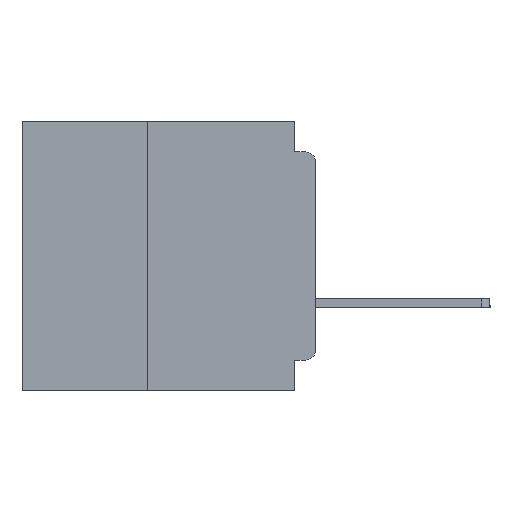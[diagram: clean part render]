
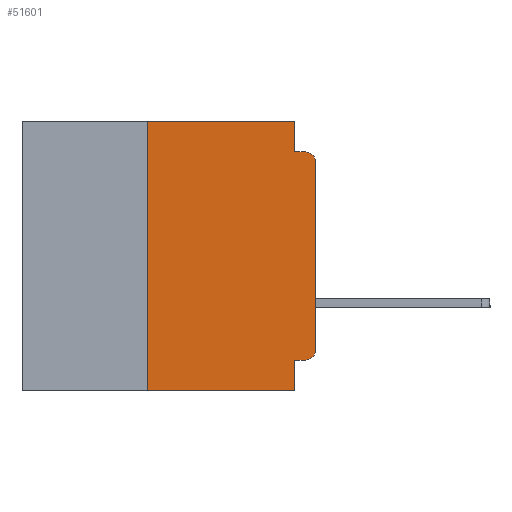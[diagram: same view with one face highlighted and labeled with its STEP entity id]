
A CAD part, left-side view. The second image highlights one B-rep face of the part: STEP entity #51601.
In plain terms, the highlighted planar face has unit normal (-1, 0, 0).
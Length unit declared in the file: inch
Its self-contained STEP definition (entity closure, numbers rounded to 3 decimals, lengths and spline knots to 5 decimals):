
#719 = CARTESIAN_POINT ( 'NONE',  ( 0., 0.031, 0. ) ) ;
#897 = LINE ( 'NONE', #25020, #22714 ) ;
#925 = EDGE_CURVE ( 'NONE', #34286, #8893, #15432, .T. ) ;
#1005 = DIRECTION ( 'NONE',  ( 0., 0., -1. ) ) ;
#1437 = ORIENTED_EDGE ( 'NONE', *, *, #4364, .F. ) ;
#3065 = LINE ( 'NONE', #24203, #42566 ) ;
#4200 = VERTEX_POINT ( 'NONE', #6494 ) ;
#4231 = ORIENTED_EDGE ( 'NONE', *, *, #51939, .F. ) ;
#4238 = DIRECTION ( 'NONE',  ( 0., -1., 0. ) ) ;
#4364 = EDGE_CURVE ( 'NONE', #16889, #38575, #39948, .T. ) ;
#4849 = CARTESIAN_POINT ( 'NONE',  ( 0., 0.031, -0.355 ) ) ;
#5773 = CARTESIAN_POINT ( 'NONE',  ( 0., 0., -0.06 ) ) ;
#6494 = CARTESIAN_POINT ( 'NONE',  ( 0., 0.015, -0.355 ) ) ;
#6663 = CARTESIAN_POINT ( 'NONE',  ( 0., 0.015, -0.06 ) ) ;
#6744 = LINE ( 'NONE', #23052, #37962 ) ;
#8608 = ORIENTED_EDGE ( 'NONE', *, *, #21193, .F. ) ;
#8769 = DIRECTION ( 'NONE',  ( 0., 0., 1. ) ) ;
#8893 = VERTEX_POINT ( 'NONE', #5773 ) ;
#9596 = CARTESIAN_POINT ( 'NONE',  ( 0., 0., 0. ) ) ;
#10766 = DIRECTION ( 'NONE',  ( 0., 0., -1. ) ) ;
#10868 = DIRECTION ( 'NONE',  ( -1., 0., 0. ) ) ;
#13558 = PLANE ( 'NONE',  #44437 ) ;
#13736 = LINE ( 'NONE', #24589, #24548 ) ;
#14921 = CIRCLE ( 'NONE', #21644, 0.015 ) ;
#15432 = LINE ( 'NONE', #9596, #22434 ) ;
#16889 = VERTEX_POINT ( 'NONE', #21702 ) ;
#17095 = VERTEX_POINT ( 'NONE', #23110 ) ;
#17670 = CARTESIAN_POINT ( 'NONE',  ( 0., 0.437, 0. ) ) ;
#17937 = ORIENTED_EDGE ( 'NONE', *, *, #28486, .F. ) ;
#19369 = CARTESIAN_POINT ( 'NONE',  ( 0., 0.25, 0. ) ) ;
#19868 = VECTOR ( 'NONE', #26842, 39.37008 ) ;
#20534 = CARTESIAN_POINT ( 'NONE',  ( 0., 0.25, -0.4 ) ) ;
#21193 = EDGE_CURVE ( 'NONE', #38575, #17095, #13736, .T. ) ;
#21644 = AXIS2_PLACEMENT_3D ( 'NONE', #35237, #10868, #39339 ) ;
#21702 = CARTESIAN_POINT ( 'NONE',  ( 0., 0.031, 0. ) ) ;
#21763 = DIRECTION ( 'NONE',  ( 1., 0., 0. ) ) ;
#22224 = ORIENTED_EDGE ( 'NONE', *, *, #41233, .T. ) ;
#22434 = VECTOR ( 'NONE', #8769, 39.37008 ) ;
#22470 = VERTEX_POINT ( 'NONE', #35575 ) ;
#22714 = VECTOR ( 'NONE', #49220, 39.37008 ) ;
#22882 = DIRECTION ( 'NONE',  ( 0., -1., 0. ) ) ;
#23052 = CARTESIAN_POINT ( 'NONE',  ( 0., 0.25, -0.4 ) ) ;
#23110 = CARTESIAN_POINT ( 'NONE',  ( 0., 0.015, -0.045 ) ) ;
#24203 = CARTESIAN_POINT ( 'NONE',  ( 0., 0., -0.355 ) ) ;
#24548 = VECTOR ( 'NONE', #4238, 39.37008 ) ;
#24589 = CARTESIAN_POINT ( 'NONE',  ( 0., 0., -0.045 ) ) ;
#25020 = CARTESIAN_POINT ( 'NONE',  ( 0., 0.437, -0.4 ) ) ;
#26067 = CARTESIAN_POINT ( 'NONE',  ( 0., 0., -0.34 ) ) ;
#26842 = DIRECTION ( 'NONE',  ( 0., 0., -1. ) ) ;
#28486 = EDGE_CURVE ( 'NONE', #35726, #16889, #41700, .T. ) ;
#28752 = VERTEX_POINT ( 'NONE', #20534 ) ;
#30394 = EDGE_CURVE ( 'NONE', #4200, #34286, #14921, .T. ) ;
#30603 = FACE_OUTER_BOUND ( 'NONE', #38740, .T. ) ;
#31379 = VERTEX_POINT ( 'NONE', #4849 ) ;
#31472 = ORIENTED_EDGE ( 'NONE', *, *, #925, .T. ) ;
#31729 = CIRCLE ( 'NONE', #39389, 0.015 ) ;
#32222 = VECTOR ( 'NONE', #22882, 39.37008 ) ;
#32594 = ORIENTED_EDGE ( 'NONE', *, *, #48910, .F. ) ;
#34286 = VERTEX_POINT ( 'NONE', #26067 ) ;
#34856 = CARTESIAN_POINT ( 'NONE',  ( 0., 0.031, -0.4 ) ) ;
#35148 = DIRECTION ( 'NONE',  ( -1., 0., 0. ) ) ;
#35237 = CARTESIAN_POINT ( 'NONE',  ( 0., 0.015, -0.34 ) ) ;
#35575 = CARTESIAN_POINT ( 'NONE',  ( 0., 0.031, -0.4 ) ) ;
#35726 = VERTEX_POINT ( 'NONE', #19369 ) ;
#37962 = VECTOR ( 'NONE', #43389, 39.37008 ) ;
#38075 = ORIENTED_EDGE ( 'NONE', *, *, #46228, .T. ) ;
#38575 = VERTEX_POINT ( 'NONE', #45020 ) ;
#38667 = VECTOR ( 'NONE', #1005, 39.37008 ) ;
#38740 = EDGE_LOOP ( 'NONE', ( #31472, #22224, #8608, #1437, #17937, #32594, #38075, #44165, #4231, #50469 ) ) ;
#39339 = DIRECTION ( 'NONE',  ( 0., 0., -1. ) ) ;
#39389 = AXIS2_PLACEMENT_3D ( 'NONE', #6663, #35148, #10766 ) ;
#39948 = LINE ( 'NONE', #719, #38667 ) ;
#40207 = DIRECTION ( 'NONE',  ( 0., 1., 0. ) ) ;
#41233 = EDGE_CURVE ( 'NONE', #8893, #17095, #31729, .T. ) ;
#41423 = LINE ( 'NONE', #34856, #19868 ) ;
#41700 = LINE ( 'NONE', #51084, #32222 ) ;
#42566 = VECTOR ( 'NONE', #40207, 39.37008 ) ;
#43389 = DIRECTION ( 'NONE',  ( 0., 0., 1. ) ) ;
#43532 = EDGE_CURVE ( 'NONE', #31379, #22470, #41423, .T. ) ;
#44165 = ORIENTED_EDGE ( 'NONE', *, *, #43532, .F. ) ;
#44437 = AXIS2_PLACEMENT_3D ( 'NONE', #17670, #21763, #50004 ) ;
#45020 = CARTESIAN_POINT ( 'NONE',  ( 0., 0.031, -0.045 ) ) ;
#46228 = EDGE_CURVE ( 'NONE', #28752, #22470, #897, .T. ) ;
#48910 = EDGE_CURVE ( 'NONE', #28752, #35726, #6744, .T. ) ;
#49220 = DIRECTION ( 'NONE',  ( 0., -1., 0. ) ) ;
#50004 = DIRECTION ( 'NONE',  ( 0., 0., -1. ) ) ;
#50469 = ORIENTED_EDGE ( 'NONE', *, *, #30394, .T. ) ;
#51084 = CARTESIAN_POINT ( 'NONE',  ( 0., 0.437, 0. ) ) ;
#51601 = ADVANCED_FACE ( 'NONE', ( #30603 ), #13558, .F. ) ;
#51939 = EDGE_CURVE ( 'NONE', #4200, #31379, #3065, .T. ) ;
